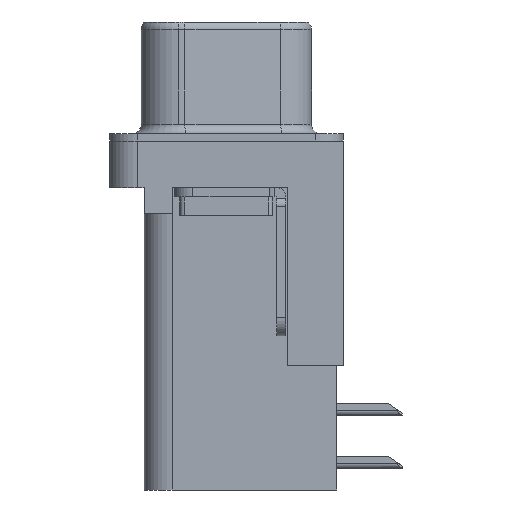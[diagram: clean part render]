
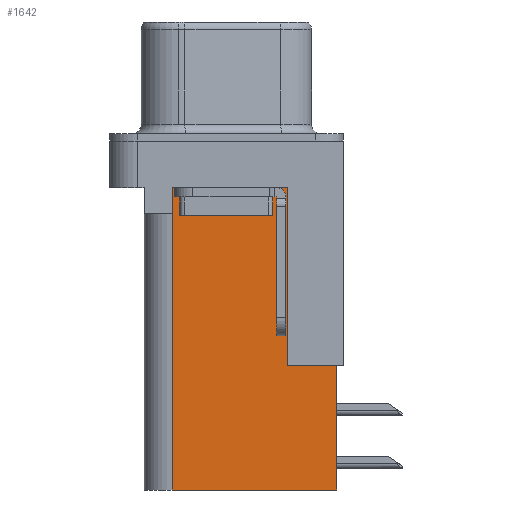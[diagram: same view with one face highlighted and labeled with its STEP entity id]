
A CAD part, left-side view. The second image highlights one B-rep face of the part: STEP entity #1642.
In plain terms, the highlighted planar face has unit normal (-1, 0, 0).
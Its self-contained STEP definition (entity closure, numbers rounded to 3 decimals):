
#78 = EDGE_CURVE ( 'NONE', #1750, #7423, #11791, .T. ) ;
#99 = VERTEX_POINT ( 'NONE', #7189 ) ;
#230 = DIRECTION ( 'NONE',  ( 0., 1., 0. ) ) ;
#390 = CARTESIAN_POINT ( 'NONE',  ( 3.765, 0., -3.9 ) ) ;
#752 = ORIENTED_EDGE ( 'NONE', *, *, #1667, .T. ) ;
#1160 = CARTESIAN_POINT ( 'NONE',  ( 3.765, -3.295, -18.76 ) ) ;
#1168 = CARTESIAN_POINT ( 'NONE',  ( 3.765, -5.925, -12.05 ) ) ;
#1360 = DIRECTION ( 'NONE',  ( 0., 1., 0. ) ) ;
#1642 = ADVANCED_FACE ( 'NONE', ( #7610 ), #15646, .F. ) ;
#1667 = EDGE_CURVE ( 'NONE', #10691, #99, #7591, .T. ) ;
#1750 = VERTEX_POINT ( 'NONE', #6083 ) ;
#2877 = DIRECTION ( 'NONE',  ( 1., 0., 0. ) ) ;
#3645 = ORIENTED_EDGE ( 'NONE', *, *, #17048, .F. ) ;
#4211 = VECTOR ( 'NONE', #18169, 1000. ) ;
#4427 = CARTESIAN_POINT ( 'NONE',  ( 3.765, -5.925, -18.76 ) ) ;
#4436 = LINE ( 'NONE', #9735, #4211 ) ;
#4566 = CARTESIAN_POINT ( 'NONE',  ( 3.765, -3.295, -2.5 ) ) ;
#4591 = VERTEX_POINT ( 'NONE', #1168 ) ;
#4701 = EDGE_CURVE ( 'NONE', #7423, #10691, #13046, .T. ) ;
#5123 = CARTESIAN_POINT ( 'NONE',  ( 3.765, 2.895, -3.9 ) ) ;
#5149 = DIRECTION ( 'NONE',  ( 0., 0., -1. ) ) ;
#5327 = EDGE_CURVE ( 'NONE', #9568, #99, #9421, .T. ) ;
#5351 = ORIENTED_EDGE ( 'NONE', *, *, #78, .T. ) ;
#5468 = ORIENTED_EDGE ( 'NONE', *, *, #5327, .F. ) ;
#6083 = CARTESIAN_POINT ( 'NONE',  ( 3.765, -3.295, -2.5 ) ) ;
#6107 = ORIENTED_EDGE ( 'NONE', *, *, #4701, .T. ) ;
#6337 = CARTESIAN_POINT ( 'NONE',  ( 3.765, 2.925, -18.76 ) ) ;
#7189 = CARTESIAN_POINT ( 'NONE',  ( 3.765, 2.925, -3.9 ) ) ;
#7423 = VERTEX_POINT ( 'NONE', #17186 ) ;
#7479 = EDGE_CURVE ( 'NONE', #4591, #11123, #15275, .T. ) ;
#7491 = VECTOR ( 'NONE', #230, 1000. ) ;
#7590 = ORIENTED_EDGE ( 'NONE', *, *, #11982, .F. ) ;
#7591 = LINE ( 'NONE', #390, #7491 ) ;
#7610 = FACE_OUTER_BOUND ( 'NONE', #12835, .T. ) ;
#7882 = ORIENTED_EDGE ( 'NONE', *, *, #17656, .T. ) ;
#8173 = AXIS2_PLACEMENT_3D ( 'NONE', #8768, #2877, #1360 ) ;
#8519 = DIRECTION ( 'NONE',  ( 0., 0., -1. ) ) ;
#8768 = CARTESIAN_POINT ( 'NONE',  ( 3.765, -3.295, -18.76 ) ) ;
#9239 = VECTOR ( 'NONE', #11824, 1000. ) ;
#9421 = LINE ( 'NONE', #11902, #9239 ) ;
#9568 = VERTEX_POINT ( 'NONE', #6337 ) ;
#9735 = CARTESIAN_POINT ( 'NONE',  ( 3.765, -3.295, -18.76 ) ) ;
#10691 = VERTEX_POINT ( 'NONE', #12278 ) ;
#11061 = VERTEX_POINT ( 'NONE', #4427 ) ;
#11123 = VERTEX_POINT ( 'NONE', #11720 ) ;
#11415 = DIRECTION ( 'NONE',  ( 0., 0., 1. ) ) ;
#11717 = VECTOR ( 'NONE', #16388, 1000. ) ;
#11720 = CARTESIAN_POINT ( 'NONE',  ( 3.765, -3.295, -12.05 ) ) ;
#11791 = LINE ( 'NONE', #4566, #11717 ) ;
#11824 = DIRECTION ( 'NONE',  ( 0., 0., 1. ) ) ;
#11902 = CARTESIAN_POINT ( 'NONE',  ( 3.765, 2.925, -18.76 ) ) ;
#11982 = EDGE_CURVE ( 'NONE', #11061, #9568, #4436, .T. ) ;
#12278 = CARTESIAN_POINT ( 'NONE',  ( 3.765, 2.895, -3.9 ) ) ;
#12835 = EDGE_LOOP ( 'NONE', ( #5351, #6107, #752, #5468, #7590, #3645, #16972, #7882 ) ) ;
#13004 = CARTESIAN_POINT ( 'NONE',  ( 3.765, -6.295, -12.05 ) ) ;
#13046 = LINE ( 'NONE', #5123, #13298 ) ;
#13298 = VECTOR ( 'NONE', #5149, 1000. ) ;
#14251 = LINE ( 'NONE', #1160, #14403 ) ;
#14403 = VECTOR ( 'NONE', #11415, 1000. ) ;
#15052 = DIRECTION ( 'NONE',  ( 0., 1., 0. ) ) ;
#15186 = VECTOR ( 'NONE', #15052, 1000. ) ;
#15275 = LINE ( 'NONE', #13004, #15186 ) ;
#15646 = PLANE ( 'NONE',  #8173 ) ;
#16388 = DIRECTION ( 'NONE',  ( 0., 1., 0. ) ) ;
#16913 = CARTESIAN_POINT ( 'NONE',  ( 3.765, -5.925, -2. ) ) ;
#16972 = ORIENTED_EDGE ( 'NONE', *, *, #7479, .T. ) ;
#17027 = VECTOR ( 'NONE', #8519, 1000. ) ;
#17048 = EDGE_CURVE ( 'NONE', #4591, #11061, #17201, .T. ) ;
#17186 = CARTESIAN_POINT ( 'NONE',  ( 3.765, 2.895, -2.5 ) ) ;
#17201 = LINE ( 'NONE', #16913, #17027 ) ;
#17656 = EDGE_CURVE ( 'NONE', #11123, #1750, #14251, .T. ) ;
#18169 = DIRECTION ( 'NONE',  ( 0., 1., 0. ) ) ;
